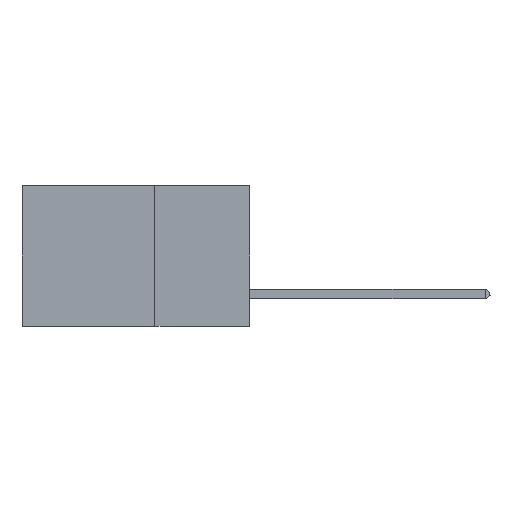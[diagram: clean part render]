
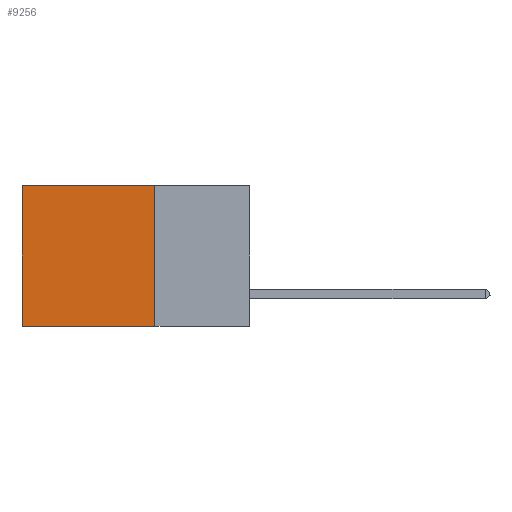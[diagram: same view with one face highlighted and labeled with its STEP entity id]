
A CAD part, left-side view. The second image highlights one B-rep face of the part: STEP entity #9256.
In plain terms, the highlighted planar face has unit normal (-1, 0, 0).
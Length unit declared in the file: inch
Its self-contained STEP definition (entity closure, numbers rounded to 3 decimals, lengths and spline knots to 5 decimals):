
#191 = EDGE_CURVE ( 'NONE', #10170, #6332, #4149, .T. ) ;
#1019 = EDGE_CURVE ( 'NONE', #1808, #6332, #19495, .T. ) ;
#1163 = EDGE_CURVE ( 'NONE', #4641, #1808, #9617, .T. ) ;
#1717 = VECTOR ( 'NONE', #17795, 39.37008 ) ;
#1808 = VERTEX_POINT ( 'NONE', #19524 ) ;
#2433 = CARTESIAN_POINT ( 'NONE',  ( 0.2875, 0.25, 0. ) ) ;
#4149 = LINE ( 'NONE', #12349, #15374 ) ;
#4641 = VERTEX_POINT ( 'NONE', #2433 ) ;
#6012 = VECTOR ( 'NONE', #11393, 39.37008 ) ;
#6044 = DIRECTION ( 'NONE',  ( 1., 0., 0. ) ) ;
#6332 = VERTEX_POINT ( 'NONE', #21364 ) ;
#6895 = DIRECTION ( 'NONE',  ( 0., 0., -1. ) ) ;
#9256 = ADVANCED_FACE ( 'NONE', ( #18150 ), #18052, .F. ) ;
#9617 = LINE ( 'NONE', #16337, #6012 ) ;
#10170 = VERTEX_POINT ( 'NONE', #11682 ) ;
#10979 = CARTESIAN_POINT ( 'NONE',  ( 0.2875, 0.25, 0. ) ) ;
#11095 = DIRECTION ( 'NONE',  ( 0., 0., -1. ) ) ;
#11393 = DIRECTION ( 'NONE',  ( 0., 1., 0. ) ) ;
#11682 = CARTESIAN_POINT ( 'NONE',  ( 0.2875, 0.25, -0.37 ) ) ;
#12147 = EDGE_CURVE ( 'NONE', #4641, #10170, #20922, .T. ) ;
#12349 = CARTESIAN_POINT ( 'NONE',  ( 0.2875, 0.25, -0.37 ) ) ;
#12719 = ORIENTED_EDGE ( 'NONE', *, *, #191, .F. ) ;
#15374 = VECTOR ( 'NONE', #21113, 39.37008 ) ;
#15428 = CARTESIAN_POINT ( 'NONE',  ( 0.2875, 0.25, 0. ) ) ;
#15460 = EDGE_LOOP ( 'NONE', ( #18337, #12719, #19647, #15643 ) ) ;
#15643 = ORIENTED_EDGE ( 'NONE', *, *, #1163, .T. ) ;
#16337 = CARTESIAN_POINT ( 'NONE',  ( 0.2875, 0.25, 0. ) ) ;
#17359 = CARTESIAN_POINT ( 'NONE',  ( 0.2875, 0.6, 0. ) ) ;
#17795 = DIRECTION ( 'NONE',  ( 0., 0., -1. ) ) ;
#18052 = PLANE ( 'NONE',  #18635 ) ;
#18150 = FACE_OUTER_BOUND ( 'NONE', #15460, .T. ) ;
#18337 = ORIENTED_EDGE ( 'NONE', *, *, #1019, .T. ) ;
#18635 = AXIS2_PLACEMENT_3D ( 'NONE', #10979, #6044, #11095 ) ;
#19495 = LINE ( 'NONE', #17359, #1717 ) ;
#19524 = CARTESIAN_POINT ( 'NONE',  ( 0.2875, 0.6, 0. ) ) ;
#19647 = ORIENTED_EDGE ( 'NONE', *, *, #12147, .F. ) ;
#20119 = VECTOR ( 'NONE', #6895, 39.37008 ) ;
#20922 = LINE ( 'NONE', #15428, #20119 ) ;
#21113 = DIRECTION ( 'NONE',  ( 0., 1., 0. ) ) ;
#21364 = CARTESIAN_POINT ( 'NONE',  ( 0.2875, 0.6, -0.37 ) ) ;
